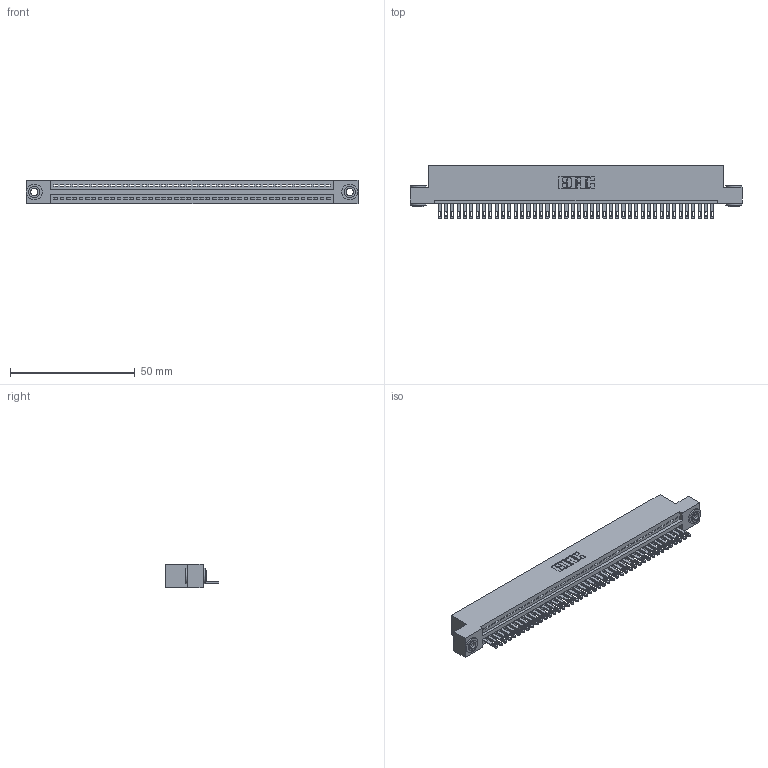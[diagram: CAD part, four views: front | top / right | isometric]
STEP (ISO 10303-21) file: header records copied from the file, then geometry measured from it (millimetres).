
FILE_DESCRIPTION (( 'STEP AP203' ), '1' );
FILE_NAME ('895-044-500-103.STEP', '2020-09-27T02:41:09', ( '' ), ( '' ), 'SwSTEP 2.0', 'SolidWorks 2020', '' );
FILE_SCHEMA (( 'CONFIG_CONTROL_DESIGN' ));
Length unit declared in the file: inch
Products named in the file (4): 845 Part_Flush Mounting Lugs - 0.156 Dia-TH; 895-044-500-103; 345-250-002_345-250-002-102; 345-292-001_345-293-100
Assembly tree (47 placements, depth 2):
  895-044-500-103
    845 Part_Flush Mounting Lugs - 0.156 Dia-TH
    345-292-001_345-293-100  x44
    345-250-002_345-250-002-102  x2
Bounding box: 132.97 x 21.51 x 9.4 mm (x, y, z)
Volume: 12692.5 mm3; surface area: 17207.7 mm2
Topology: 47 solids, 47 shells, 2540 faces, 7809 edges, 5202 vertices
Faces by surface type: plane 1586, cylinder 946, cone 8
Entity records: 33426 total; most frequent: CARTESIAN_POINT 5767, ORIENTED_EDGE 5738, DIRECTION 5067, EDGE_CURVE 2869, VECTOR 2533, LINE 2533, VERTEX_POINT 1910, AXIS2_PLACEMENT_3D 1267
